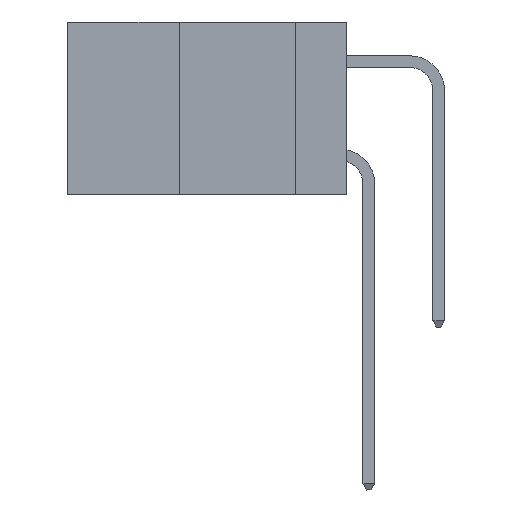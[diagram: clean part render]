
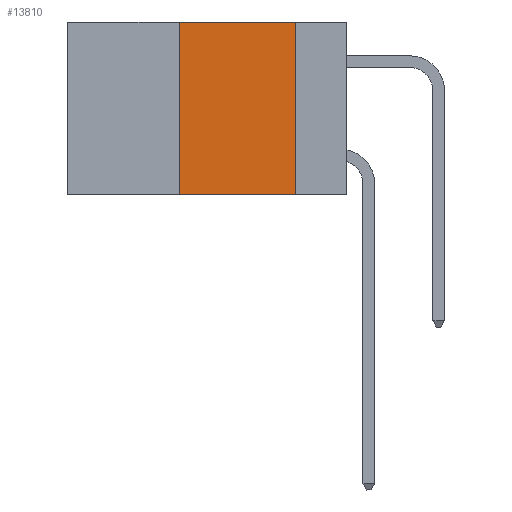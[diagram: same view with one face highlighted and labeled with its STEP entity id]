
A CAD part, left-side view. The second image highlights one B-rep face of the part: STEP entity #13810.
In plain terms, the highlighted planar face has unit normal (-1, 0, 0).
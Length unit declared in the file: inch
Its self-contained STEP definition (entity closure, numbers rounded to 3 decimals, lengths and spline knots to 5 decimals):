
#234 = CARTESIAN_POINT ( 'NONE',  ( 0., 0.11, 0. ) ) ;
#1449 = DIRECTION ( 'NONE',  ( 0., 0., 1. ) ) ;
#1610 = EDGE_CURVE ( 'NONE', #11663, #18738, #6192, .T. ) ;
#1800 = DIRECTION ( 'NONE',  ( 1., 0., 0. ) ) ;
#1915 = CARTESIAN_POINT ( 'NONE',  ( 0., 0.11, -0.37 ) ) ;
#2078 = VECTOR ( 'NONE', #6550, 39.37008 ) ;
#2571 = VECTOR ( 'NONE', #17079, 39.37008 ) ;
#3031 = LINE ( 'NONE', #5770, #11213 ) ;
#3118 = ORIENTED_EDGE ( 'NONE', *, *, #1610, .T. ) ;
#3623 = ORIENTED_EDGE ( 'NONE', *, *, #14609, .F. ) ;
#3704 = EDGE_CURVE ( 'NONE', #9993, #18738, #3031, .T. ) ;
#5601 = VECTOR ( 'NONE', #1449, 39.37008 ) ;
#5770 = CARTESIAN_POINT ( 'NONE',  ( 0., 0.11, 0. ) ) ;
#6136 = DIRECTION ( 'NONE',  ( 0., 0., -1. ) ) ;
#6192 = LINE ( 'NONE', #18133, #2571 ) ;
#6441 = EDGE_LOOP ( 'NONE', ( #12255, #3623, #7201, #3118 ) ) ;
#6550 = DIRECTION ( 'NONE',  ( 0., -1., 0. ) ) ;
#7201 = ORIENTED_EDGE ( 'NONE', *, *, #16012, .F. ) ;
#7386 = FACE_OUTER_BOUND ( 'NONE', #6441, .T. ) ;
#8672 = CARTESIAN_POINT ( 'NONE',  ( 0., 0.36, -0.37 ) ) ;
#9993 = VERTEX_POINT ( 'NONE', #234 ) ;
#10016 = CARTESIAN_POINT ( 'NONE',  ( 0., 0.36, 0. ) ) ;
#10670 = CARTESIAN_POINT ( 'NONE',  ( 0., 0.36, 0. ) ) ;
#10998 = CARTESIAN_POINT ( 'NONE',  ( 0., 0.6, 0. ) ) ;
#11213 = VECTOR ( 'NONE', #6136, 39.37008 ) ;
#11663 = VERTEX_POINT ( 'NONE', #8672 ) ;
#12255 = ORIENTED_EDGE ( 'NONE', *, *, #3704, .F. ) ;
#12468 = PLANE ( 'NONE',  #15924 ) ;
#12538 = DIRECTION ( 'NONE',  ( 0., 0., -1. ) ) ;
#12705 = CARTESIAN_POINT ( 'NONE',  ( 0., 0.6, 0. ) ) ;
#13760 = LINE ( 'NONE', #10670, #5601 ) ;
#13810 = ADVANCED_FACE ( 'NONE', ( #7386 ), #12468, .F. ) ;
#14609 = EDGE_CURVE ( 'NONE', #17622, #9993, #18320, .T. ) ;
#15924 = AXIS2_PLACEMENT_3D ( 'NONE', #10998, #1800, #12538 ) ;
#16012 = EDGE_CURVE ( 'NONE', #11663, #17622, #13760, .T. ) ;
#17079 = DIRECTION ( 'NONE',  ( 0., -1., 0. ) ) ;
#17622 = VERTEX_POINT ( 'NONE', #10016 ) ;
#18133 = CARTESIAN_POINT ( 'NONE',  ( 0., 0.6, -0.37 ) ) ;
#18320 = LINE ( 'NONE', #12705, #2078 ) ;
#18738 = VERTEX_POINT ( 'NONE', #1915 ) ;
